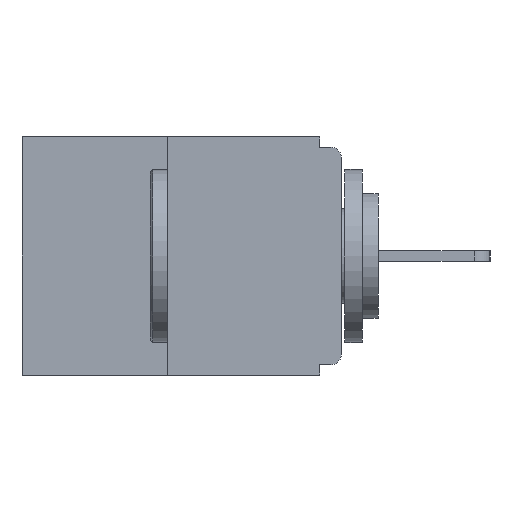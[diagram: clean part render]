
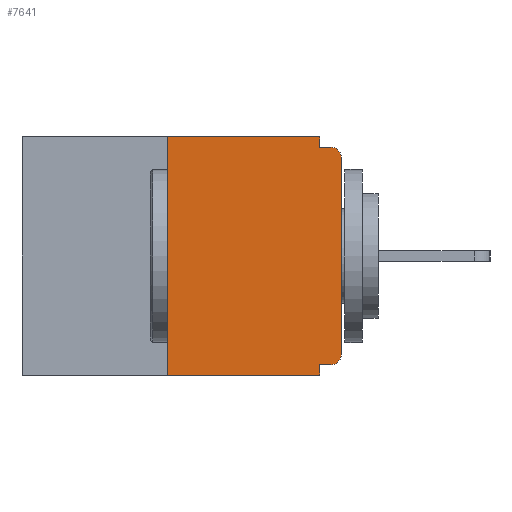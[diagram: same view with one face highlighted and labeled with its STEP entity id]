
A CAD part, left-side view. The second image highlights one B-rep face of the part: STEP entity #7641.
In plain terms, the highlighted planar face has unit normal (-1, 0, 0).
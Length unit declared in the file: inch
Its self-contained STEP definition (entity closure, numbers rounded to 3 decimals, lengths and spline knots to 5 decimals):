
#236 = EDGE_CURVE ( 'NONE', #12381, #5504, #19196, .T. ) ;
#700 = VECTOR ( 'NONE', #1130, 39.37008 ) ;
#723 = CARTESIAN_POINT ( 'NONE',  ( 0., 0.015, -0.015 ) ) ;
#763 = CARTESIAN_POINT ( 'NONE',  ( 0., 0.031, -0.343 ) ) ;
#813 = VECTOR ( 'NONE', #26065, 39.37008 ) ;
#831 = VERTEX_POINT ( 'NONE', #6540 ) ;
#1130 = DIRECTION ( 'NONE',  ( 0., -1., 0. ) ) ;
#1334 = VECTOR ( 'NONE', #17410, 39.37008 ) ;
#1442 = DIRECTION ( 'NONE',  ( 1., 0., 0. ) ) ;
#1447 = ORIENTED_EDGE ( 'NONE', *, *, #236, .T. ) ;
#1475 = CARTESIAN_POINT ( 'NONE',  ( 0., 0.015, -0.03 ) ) ;
#2527 = LINE ( 'NONE', #6703, #12417 ) ;
#2733 = EDGE_CURVE ( 'NONE', #6909, #23251, #11216, .T. ) ;
#3053 = CARTESIAN_POINT ( 'NONE',  ( 0., 0.46, 0. ) ) ;
#4288 = CARTESIAN_POINT ( 'NONE',  ( 0., 0.031, -0.343 ) ) ;
#4573 = CARTESIAN_POINT ( 'NONE',  ( 0., 0.015, -0.328 ) ) ;
#5149 = LINE ( 'NONE', #5288, #17243 ) ;
#5151 = CARTESIAN_POINT ( 'NONE',  ( 0., 0.46, 0. ) ) ;
#5288 = CARTESIAN_POINT ( 'NONE',  ( 0., 0., -0.015 ) ) ;
#5344 = ORIENTED_EDGE ( 'NONE', *, *, #13822, .F. ) ;
#5490 = EDGE_CURVE ( 'NONE', #6193, #5504, #5149, .T. ) ;
#5504 = VERTEX_POINT ( 'NONE', #723 ) ;
#5560 = CARTESIAN_POINT ( 'NONE',  ( 0., 0.25, 0. ) ) ;
#6031 = VERTEX_POINT ( 'NONE', #18334 ) ;
#6193 = VERTEX_POINT ( 'NONE', #16738 ) ;
#6540 = CARTESIAN_POINT ( 'NONE',  ( 0., 0.25, -0.343 ) ) ;
#6703 = CARTESIAN_POINT ( 'NONE',  ( 0., 0., 0. ) ) ;
#6868 = EDGE_CURVE ( 'NONE', #11456, #25988, #16278, .T. ) ;
#6909 = VERTEX_POINT ( 'NONE', #5560 ) ;
#7207 = DIRECTION ( 'NONE',  ( 0., 0., 1. ) ) ;
#7641 = ADVANCED_FACE ( 'NONE', ( #23730 ), #21442, .F. ) ;
#8377 = VECTOR ( 'NONE', #16149, 39.37008 ) ;
#9610 = CARTESIAN_POINT ( 'NONE',  ( 0., 0.46, -0.343 ) ) ;
#9950 = VECTOR ( 'NONE', #17649, 39.37008 ) ;
#10585 = EDGE_CURVE ( 'NONE', #6031, #12381, #2527, .T. ) ;
#10815 = AXIS2_PLACEMENT_3D ( 'NONE', #23138, #22599, #14818 ) ;
#10841 = VECTOR ( 'NONE', #14504, 39.37008 ) ;
#11033 = ORIENTED_EDGE ( 'NONE', *, *, #24397, .T. ) ;
#11216 = LINE ( 'NONE', #5151, #700 ) ;
#11444 = AXIS2_PLACEMENT_3D ( 'NONE', #3053, #1442, #17808 ) ;
#11456 = VERTEX_POINT ( 'NONE', #4573 ) ;
#11502 = LINE ( 'NONE', #9610, #9950 ) ;
#11816 = DIRECTION ( 'NONE',  ( -1., 0., 0. ) ) ;
#12381 = VERTEX_POINT ( 'NONE', #12600 ) ;
#12417 = VECTOR ( 'NONE', #7207, 39.37008 ) ;
#12600 = CARTESIAN_POINT ( 'NONE',  ( 0., 0., -0.03 ) ) ;
#12975 = ORIENTED_EDGE ( 'NONE', *, *, #10585, .T. ) ;
#13332 = LINE ( 'NONE', #21782, #813 ) ;
#13713 = ORIENTED_EDGE ( 'NONE', *, *, #5490, .F. ) ;
#13822 = EDGE_CURVE ( 'NONE', #831, #6909, #21172, .T. ) ;
#14377 = EDGE_CURVE ( 'NONE', #831, #21316, #11502, .T. ) ;
#14504 = DIRECTION ( 'NONE',  ( 0., 0., -1. ) ) ;
#14818 = DIRECTION ( 'NONE',  ( 0., 0., -1. ) ) ;
#16149 = DIRECTION ( 'NONE',  ( 0., 1., 0. ) ) ;
#16157 = CARTESIAN_POINT ( 'NONE',  ( 0., 0.031, -0.328 ) ) ;
#16278 = LINE ( 'NONE', #22067, #8377 ) ;
#16738 = CARTESIAN_POINT ( 'NONE',  ( 0., 0.031, -0.015 ) ) ;
#17243 = VECTOR ( 'NONE', #21266, 39.37008 ) ;
#17410 = DIRECTION ( 'NONE',  ( 0., 0., 1. ) ) ;
#17649 = DIRECTION ( 'NONE',  ( 0., -1., 0. ) ) ;
#17808 = DIRECTION ( 'NONE',  ( 0., 0., -1. ) ) ;
#18334 = CARTESIAN_POINT ( 'NONE',  ( 0., 0., -0.313 ) ) ;
#18717 = ORIENTED_EDGE ( 'NONE', *, *, #19936, .F. ) ;
#19196 = CIRCLE ( 'NONE', #24356, 0.015 ) ;
#19342 = CIRCLE ( 'NONE', #10815, 0.015 ) ;
#19345 = CARTESIAN_POINT ( 'NONE',  ( 0., 0.031, 0. ) ) ;
#19936 = EDGE_CURVE ( 'NONE', #23251, #6193, #13332, .T. ) ;
#20313 = ORIENTED_EDGE ( 'NONE', *, *, #6868, .F. ) ;
#20513 = ORIENTED_EDGE ( 'NONE', *, *, #2733, .F. ) ;
#20552 = ORIENTED_EDGE ( 'NONE', *, *, #24562, .F. ) ;
#21172 = LINE ( 'NONE', #23193, #1334 ) ;
#21201 = ORIENTED_EDGE ( 'NONE', *, *, #14377, .T. ) ;
#21266 = DIRECTION ( 'NONE',  ( 0., -1., 0. ) ) ;
#21316 = VERTEX_POINT ( 'NONE', #763 ) ;
#21442 = PLANE ( 'NONE',  #11444 ) ;
#21782 = CARTESIAN_POINT ( 'NONE',  ( 0., 0.031, 0. ) ) ;
#22067 = CARTESIAN_POINT ( 'NONE',  ( 0., 0., -0.328 ) ) ;
#22081 = EDGE_LOOP ( 'NONE', ( #20513, #5344, #21201, #20552, #20313, #11033, #12975, #1447, #13713, #18717 ) ) ;
#22599 = DIRECTION ( 'NONE',  ( -1., 0., 0. ) ) ;
#23090 = LINE ( 'NONE', #4288, #10841 ) ;
#23138 = CARTESIAN_POINT ( 'NONE',  ( 0., 0.015, -0.313 ) ) ;
#23193 = CARTESIAN_POINT ( 'NONE',  ( 0., 0.25, 0. ) ) ;
#23251 = VERTEX_POINT ( 'NONE', #19345 ) ;
#23730 = FACE_OUTER_BOUND ( 'NONE', #22081, .T. ) ;
#24356 = AXIS2_PLACEMENT_3D ( 'NONE', #1475, #11816, #26034 ) ;
#24397 = EDGE_CURVE ( 'NONE', #11456, #6031, #19342, .T. ) ;
#24562 = EDGE_CURVE ( 'NONE', #25988, #21316, #23090, .T. ) ;
#25988 = VERTEX_POINT ( 'NONE', #16157 ) ;
#26034 = DIRECTION ( 'NONE',  ( 0., 0., -1. ) ) ;
#26065 = DIRECTION ( 'NONE',  ( 0., 0., -1. ) ) ;
